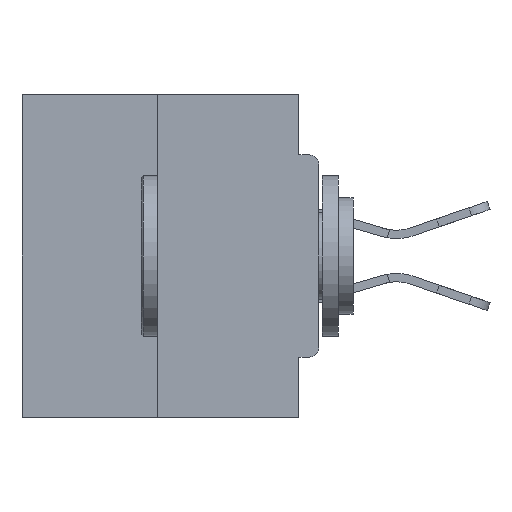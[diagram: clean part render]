
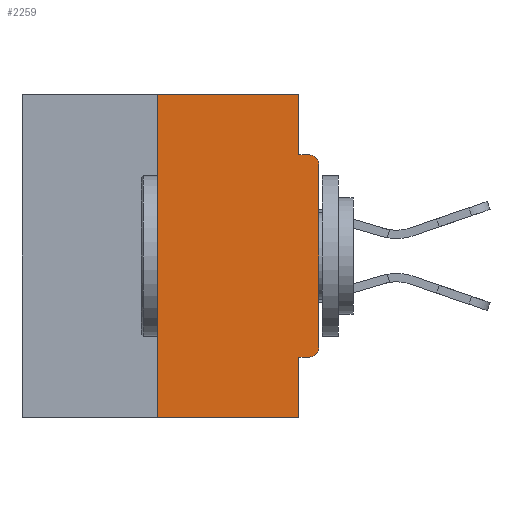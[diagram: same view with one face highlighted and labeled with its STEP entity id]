
A CAD part, left-side view. The second image highlights one B-rep face of the part: STEP entity #2259.
In plain terms, the highlighted planar face has unit normal (-1, 0, 0).
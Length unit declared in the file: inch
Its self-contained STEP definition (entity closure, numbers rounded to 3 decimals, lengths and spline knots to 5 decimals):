
#988 = CARTESIAN_POINT ( 'NONE',  ( 0., 0.031, 0. ) ) ;
#1406 = EDGE_LOOP ( 'NONE', ( #6407, #5701, #3128, #8074, #8273, #34079, #2075, #32918, #25891, #29432 ) ) ;
#1447 = LINE ( 'NONE', #20871, #16437 ) ;
#1589 = DIRECTION ( 'NONE',  ( 0., 0., 1. ) ) ;
#2030 = LINE ( 'NONE', #988, #9956 ) ;
#2075 = ORIENTED_EDGE ( 'NONE', *, *, #36133, .T. ) ;
#2259 = ADVANCED_FACE ( 'NONE', ( #4523 ), #21019, .F. ) ;
#2545 = DIRECTION ( 'NONE',  ( 0., -1., 0. ) ) ;
#3128 = ORIENTED_EDGE ( 'NONE', *, *, #34535, .T. ) ;
#4094 = CARTESIAN_POINT ( 'NONE',  ( 0., 0.015, -0.0935 ) ) ;
#4097 = VERTEX_POINT ( 'NONE', #15718 ) ;
#4245 = CARTESIAN_POINT ( 'NONE',  ( 0., 0.015, -0.1085 ) ) ;
#4329 = VECTOR ( 'NONE', #1589, 39.37008 ) ;
#4523 = FACE_OUTER_BOUND ( 'NONE', #1406, .T. ) ;
#4524 = VECTOR ( 'NONE', #31420, 39.37008 ) ;
#5701 = ORIENTED_EDGE ( 'NONE', *, *, #32302, .F. ) ;
#5958 = VERTEX_POINT ( 'NONE', #22599 ) ;
#6407 = ORIENTED_EDGE ( 'NONE', *, *, #8501, .F. ) ;
#7026 = VERTEX_POINT ( 'NONE', #31385 ) ;
#7309 = VERTEX_POINT ( 'NONE', #4094 ) ;
#8074 = ORIENTED_EDGE ( 'NONE', *, *, #18282, .F. ) ;
#8273 = ORIENTED_EDGE ( 'NONE', *, *, #8612, .F. ) ;
#8501 = EDGE_CURVE ( 'NONE', #4097, #5958, #1447, .T. ) ;
#8612 = EDGE_CURVE ( 'NONE', #25190, #7026, #12013, .T. ) ;
#9424 = DIRECTION ( 'NONE',  ( 0., 0., -1. ) ) ;
#9898 = CARTESIAN_POINT ( 'NONE',  ( 0., 0.031, -0.5 ) ) ;
#9956 = VECTOR ( 'NONE', #18361, 39.37008 ) ;
#10454 = CARTESIAN_POINT ( 'NONE',  ( 0., 0.031, -0.5 ) ) ;
#10833 = LINE ( 'NONE', #9898, #12193 ) ;
#11256 = CARTESIAN_POINT ( 'NONE',  ( 0., 0.031, -0.0935 ) ) ;
#11355 = CARTESIAN_POINT ( 'NONE',  ( 0., 0., -0.4065 ) ) ;
#12013 = LINE ( 'NONE', #11355, #4524 ) ;
#12193 = VECTOR ( 'NONE', #18311, 39.37008 ) ;
#12417 = VECTOR ( 'NONE', #27428, 39.37008 ) ;
#12490 = DIRECTION ( 'NONE',  ( 0., 0., -1. ) ) ;
#12513 = CARTESIAN_POINT ( 'NONE',  ( 0., 0.46, 0. ) ) ;
#12778 = DIRECTION ( 'NONE',  ( -1., 0., 0. ) ) ;
#13488 = CARTESIAN_POINT ( 'NONE',  ( 0., 0.46, -0.5 ) ) ;
#14743 = CARTESIAN_POINT ( 'NONE',  ( 0., 0., -0.1085 ) ) ;
#15361 = LINE ( 'NONE', #35141, #4329 ) ;
#15576 = EDGE_CURVE ( 'NONE', #25190, #21349, #32776, .T. ) ;
#15718 = CARTESIAN_POINT ( 'NONE',  ( 0., 0.25, 0. ) ) ;
#16277 = VERTEX_POINT ( 'NONE', #28553 ) ;
#16437 = VECTOR ( 'NONE', #21235, 39.37008 ) ;
#17320 = EDGE_CURVE ( 'NONE', #33457, #7309, #34765, .T. ) ;
#18248 = AXIS2_PLACEMENT_3D ( 'NONE', #4245, #26518, #12490 ) ;
#18282 = EDGE_CURVE ( 'NONE', #7026, #36194, #10833, .T. ) ;
#18311 = DIRECTION ( 'NONE',  ( 0., 0., -1. ) ) ;
#18361 = DIRECTION ( 'NONE',  ( 0., 0., -1. ) ) ;
#18474 = DIRECTION ( 'NONE',  ( 0., -1., 0. ) ) ;
#20871 = CARTESIAN_POINT ( 'NONE',  ( 0., 0.46, 0. ) ) ;
#21019 = PLANE ( 'NONE',  #24167 ) ;
#21084 = AXIS2_PLACEMENT_3D ( 'NONE', #29393, #12778, #9424 ) ;
#21123 = CARTESIAN_POINT ( 'NONE',  ( 0., 0.015, -0.4065 ) ) ;
#21172 = CARTESIAN_POINT ( 'NONE',  ( 0., 0., -0.0935 ) ) ;
#21235 = DIRECTION ( 'NONE',  ( 0., -1., 0. ) ) ;
#21349 = VERTEX_POINT ( 'NONE', #35494 ) ;
#21646 = EDGE_CURVE ( 'NONE', #34211, #7309, #31725, .T. ) ;
#22599 = CARTESIAN_POINT ( 'NONE',  ( 0., 0.031, 0. ) ) ;
#23467 = DIRECTION ( 'NONE',  ( 1., 0., 0. ) ) ;
#23562 = VECTOR ( 'NONE', #2545, 39.37008 ) ;
#24167 = AXIS2_PLACEMENT_3D ( 'NONE', #12513, #23467, #29144 ) ;
#24593 = VECTOR ( 'NONE', #18474, 39.37008 ) ;
#25190 = VERTEX_POINT ( 'NONE', #21123 ) ;
#25891 = ORIENTED_EDGE ( 'NONE', *, *, #17320, .F. ) ;
#26518 = DIRECTION ( 'NONE',  ( -1., 0., 0. ) ) ;
#27172 = CARTESIAN_POINT ( 'NONE',  ( 0., 0., 0. ) ) ;
#27428 = DIRECTION ( 'NONE',  ( 0., 0., 1. ) ) ;
#28553 = CARTESIAN_POINT ( 'NONE',  ( 0., 0.25, -0.5 ) ) ;
#29144 = DIRECTION ( 'NONE',  ( 0., 0., -1. ) ) ;
#29167 = LINE ( 'NONE', #27172, #12417 ) ;
#29393 = CARTESIAN_POINT ( 'NONE',  ( 0., 0.015, -0.3915 ) ) ;
#29432 = ORIENTED_EDGE ( 'NONE', *, *, #33893, .F. ) ;
#30197 = LINE ( 'NONE', #13488, #23562 ) ;
#31385 = CARTESIAN_POINT ( 'NONE',  ( 0., 0.031, -0.4065 ) ) ;
#31420 = DIRECTION ( 'NONE',  ( 0., 1., 0. ) ) ;
#31725 = CIRCLE ( 'NONE', #18248, 0.015 ) ;
#32302 = EDGE_CURVE ( 'NONE', #16277, #4097, #15361, .T. ) ;
#32776 = CIRCLE ( 'NONE', #21084, 0.015 ) ;
#32918 = ORIENTED_EDGE ( 'NONE', *, *, #21646, .T. ) ;
#33457 = VERTEX_POINT ( 'NONE', #11256 ) ;
#33893 = EDGE_CURVE ( 'NONE', #5958, #33457, #2030, .T. ) ;
#34079 = ORIENTED_EDGE ( 'NONE', *, *, #15576, .T. ) ;
#34211 = VERTEX_POINT ( 'NONE', #14743 ) ;
#34535 = EDGE_CURVE ( 'NONE', #16277, #36194, #30197, .T. ) ;
#34765 = LINE ( 'NONE', #21172, #24593 ) ;
#35141 = CARTESIAN_POINT ( 'NONE',  ( 0., 0.25, 0. ) ) ;
#35494 = CARTESIAN_POINT ( 'NONE',  ( 0., 0., -0.3915 ) ) ;
#36133 = EDGE_CURVE ( 'NONE', #21349, #34211, #29167, .T. ) ;
#36194 = VERTEX_POINT ( 'NONE', #10454 ) ;
